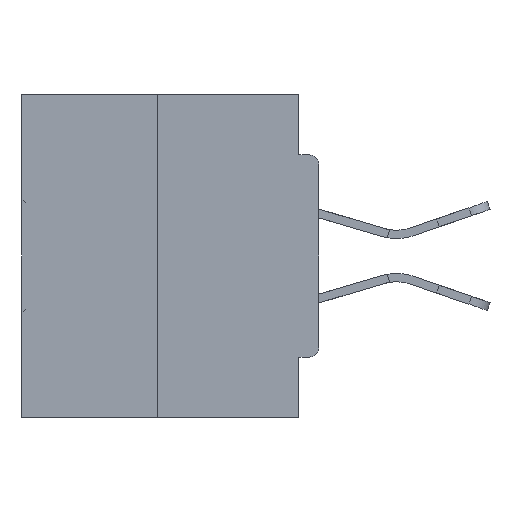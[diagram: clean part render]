
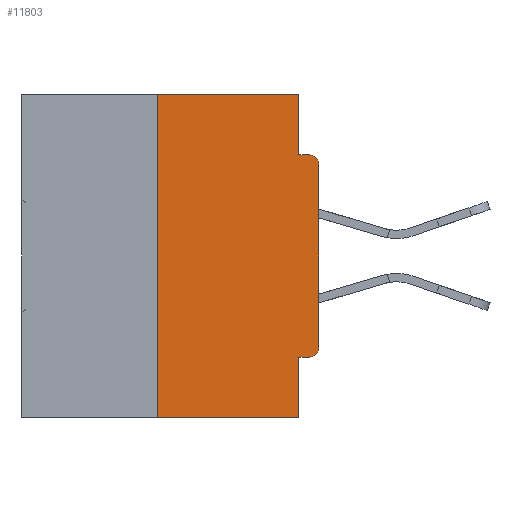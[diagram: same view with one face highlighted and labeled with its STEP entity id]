
A CAD part, left-side view. The second image highlights one B-rep face of the part: STEP entity #11803.
In plain terms, the highlighted planar face has unit normal (-1, 0, 0).
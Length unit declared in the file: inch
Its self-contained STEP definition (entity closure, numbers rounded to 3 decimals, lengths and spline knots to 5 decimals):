
#27 = EDGE_LOOP ( 'NONE', ( #44541, #1529, #10875, #34296, #3236, #12802, #28808, #5405, #10041, #44194 ) ) ;
#261 = VERTEX_POINT ( 'NONE', #5652 ) ;
#847 = CARTESIAN_POINT ( 'NONE',  ( 0., 0.031, -0.0935 ) ) ;
#1048 = EDGE_CURVE ( 'NONE', #7537, #20547, #39851, .T. ) ;
#1529 = ORIENTED_EDGE ( 'NONE', *, *, #31859, .F. ) ;
#1756 = VERTEX_POINT ( 'NONE', #32750 ) ;
#2447 = CARTESIAN_POINT ( 'NONE',  ( 0., 0.015, -0.3915 ) ) ;
#2871 = LINE ( 'NONE', #11822, #10491 ) ;
#3210 = VECTOR ( 'NONE', #13479, 39.37008 ) ;
#3236 = ORIENTED_EDGE ( 'NONE', *, *, #12570, .F. ) ;
#3368 = LINE ( 'NONE', #19658, #37310 ) ;
#4573 = VERTEX_POINT ( 'NONE', #27012 ) ;
#5405 = ORIENTED_EDGE ( 'NONE', *, *, #20203, .T. ) ;
#5652 = CARTESIAN_POINT ( 'NONE',  ( 0., 0.031, -0.4065 ) ) ;
#6066 = DIRECTION ( 'NONE',  ( -1., 0., 0. ) ) ;
#7537 = VERTEX_POINT ( 'NONE', #31702 ) ;
#8873 = AXIS2_PLACEMENT_3D ( 'NONE', #23132, #23574, #20578 ) ;
#10041 = ORIENTED_EDGE ( 'NONE', *, *, #17004, .F. ) ;
#10451 = CARTESIAN_POINT ( 'NONE',  ( 0., 0., 0. ) ) ;
#10491 = VECTOR ( 'NONE', #33380, 39.37008 ) ;
#10875 = ORIENTED_EDGE ( 'NONE', *, *, #1048, .T. ) ;
#10904 = EDGE_CURVE ( 'NONE', #261, #20547, #42771, .T. ) ;
#11803 = ADVANCED_FACE ( 'NONE', ( #20190 ), #44434, .F. ) ;
#11822 = CARTESIAN_POINT ( 'NONE',  ( 0., 0., -0.4065 ) ) ;
#12570 = EDGE_CURVE ( 'NONE', #17003, #261, #2871, .T. ) ;
#12615 = DIRECTION ( 'NONE',  ( 0., 0., -1. ) ) ;
#12802 = ORIENTED_EDGE ( 'NONE', *, *, #27866, .T. ) ;
#13129 = VECTOR ( 'NONE', #37961, 39.37008 ) ;
#13232 = CARTESIAN_POINT ( 'NONE',  ( 0., 0.46, 0. ) ) ;
#13479 = DIRECTION ( 'NONE',  ( 0., 0., 1. ) ) ;
#13841 = DIRECTION ( 'NONE',  ( 1., 0., 0. ) ) ;
#13949 = CARTESIAN_POINT ( 'NONE',  ( 0., 0.25, 0. ) ) ;
#14518 = CARTESIAN_POINT ( 'NONE',  ( 0., 0.031, -0.5 ) ) ;
#14746 = EDGE_CURVE ( 'NONE', #1756, #36008, #3368, .T. ) ;
#15123 = DIRECTION ( 'NONE',  ( 0., 0., -1. ) ) ;
#15423 = CARTESIAN_POINT ( 'NONE',  ( 0., 0.46, -0.5 ) ) ;
#17003 = VERTEX_POINT ( 'NONE', #42711 ) ;
#17004 = EDGE_CURVE ( 'NONE', #26590, #28642, #38706, .T. ) ;
#17248 = VECTOR ( 'NONE', #26870, 39.37008 ) ;
#17304 = LINE ( 'NONE', #10451, #3210 ) ;
#18745 = DIRECTION ( 'NONE',  ( 0., -1., 0. ) ) ;
#19658 = CARTESIAN_POINT ( 'NONE',  ( 0., 0.46, 0. ) ) ;
#19962 = DIRECTION ( 'NONE',  ( 0., -1., 0. ) ) ;
#20190 = FACE_OUTER_BOUND ( 'NONE', #27, .T. ) ;
#20203 = EDGE_CURVE ( 'NONE', #38919, #28642, #21680, .T. ) ;
#20547 = VERTEX_POINT ( 'NONE', #27237 ) ;
#20578 = DIRECTION ( 'NONE',  ( 0., 0., -1. ) ) ;
#21680 = CIRCLE ( 'NONE', #8873, 0.015 ) ;
#22494 = CARTESIAN_POINT ( 'NONE',  ( 0., 0.015, -0.0935 ) ) ;
#23132 = CARTESIAN_POINT ( 'NONE',  ( 0., 0.015, -0.1085 ) ) ;
#23450 = CARTESIAN_POINT ( 'NONE',  ( 0., 0.031, 0. ) ) ;
#23544 = DIRECTION ( 'NONE',  ( 0., -1., 0. ) ) ;
#23574 = DIRECTION ( 'NONE',  ( -1., 0., 0. ) ) ;
#24574 = VECTOR ( 'NONE', #15123, 39.37008 ) ;
#26590 = VERTEX_POINT ( 'NONE', #847 ) ;
#26870 = DIRECTION ( 'NONE',  ( 0., 0., -1. ) ) ;
#27012 = CARTESIAN_POINT ( 'NONE',  ( 0., 0., -0.3915 ) ) ;
#27237 = CARTESIAN_POINT ( 'NONE',  ( 0., 0.031, -0.5 ) ) ;
#27421 = LINE ( 'NONE', #23450, #17248 ) ;
#27866 = EDGE_CURVE ( 'NONE', #17003, #4573, #36741, .T. ) ;
#28642 = VERTEX_POINT ( 'NONE', #22494 ) ;
#28808 = ORIENTED_EDGE ( 'NONE', *, *, #33343, .T. ) ;
#29479 = CARTESIAN_POINT ( 'NONE',  ( 0., 0.031, 0. ) ) ;
#30874 = LINE ( 'NONE', #13949, #13129 ) ;
#30880 = EDGE_CURVE ( 'NONE', #36008, #26590, #27421, .T. ) ;
#31702 = CARTESIAN_POINT ( 'NONE',  ( 0., 0.25, -0.5 ) ) ;
#31859 = EDGE_CURVE ( 'NONE', #7537, #1756, #30874, .T. ) ;
#32750 = CARTESIAN_POINT ( 'NONE',  ( 0., 0.25, 0. ) ) ;
#33343 = EDGE_CURVE ( 'NONE', #4573, #38919, #17304, .T. ) ;
#33380 = DIRECTION ( 'NONE',  ( 0., 1., 0. ) ) ;
#34296 = ORIENTED_EDGE ( 'NONE', *, *, #10904, .F. ) ;
#34757 = AXIS2_PLACEMENT_3D ( 'NONE', #2447, #6066, #12615 ) ;
#36008 = VERTEX_POINT ( 'NONE', #29479 ) ;
#36104 = VECTOR ( 'NONE', #18745, 39.37008 ) ;
#36584 = CARTESIAN_POINT ( 'NONE',  ( 0., 0., -0.0935 ) ) ;
#36741 = CIRCLE ( 'NONE', #34757, 0.015 ) ;
#37277 = DIRECTION ( 'NONE',  ( 0., 0., -1. ) ) ;
#37310 = VECTOR ( 'NONE', #19962, 39.37008 ) ;
#37610 = VECTOR ( 'NONE', #23544, 39.37008 ) ;
#37961 = DIRECTION ( 'NONE',  ( 0., 0., 1. ) ) ;
#38706 = LINE ( 'NONE', #36584, #37610 ) ;
#38919 = VERTEX_POINT ( 'NONE', #40624 ) ;
#39851 = LINE ( 'NONE', #15423, #36104 ) ;
#40624 = CARTESIAN_POINT ( 'NONE',  ( 0., 0., -0.1085 ) ) ;
#42711 = CARTESIAN_POINT ( 'NONE',  ( 0., 0.015, -0.4065 ) ) ;
#42771 = LINE ( 'NONE', #14518, #24574 ) ;
#44194 = ORIENTED_EDGE ( 'NONE', *, *, #30880, .F. ) ;
#44316 = AXIS2_PLACEMENT_3D ( 'NONE', #13232, #13841, #37277 ) ;
#44434 = PLANE ( 'NONE',  #44316 ) ;
#44541 = ORIENTED_EDGE ( 'NONE', *, *, #14746, .F. ) ;
